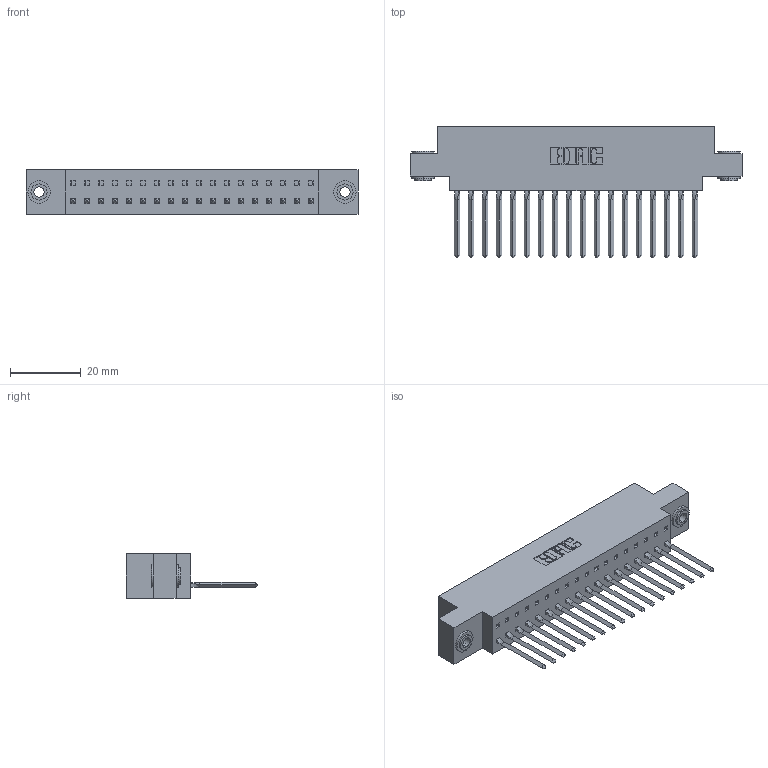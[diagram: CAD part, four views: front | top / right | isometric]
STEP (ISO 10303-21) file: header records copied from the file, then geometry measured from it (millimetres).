
FILE_DESCRIPTION (( 'STEP AP203' ), '1' );
FILE_NAME ('317-018-541-603.STEP', '2020-02-27T15:54:17', ( '' ), ( '' ), 'SwSTEP 2.0', 'SolidWorks 2016', '' );
FILE_SCHEMA (( 'CONFIG_CONTROL_DESIGN' ));
Length unit declared in the file: inch
Products named in the file (4): 317-290-002_541; 345-250-002_345-250-002-102; 317 Part_.156 Dia - TH; 317-018-541-603
Assembly tree (21 placements, depth 2):
  317-018-541-603
    317 Part_.156 Dia - TH
    317-290-002_541  x18
    345-250-002_345-250-002-102  x2
Bounding box: 94.03 x 37.34 x 12.7 mm (x, y, z)
Volume: 14530.1 mm3; surface area: 19946.5 mm2
Topology: 21 solids, 21 shells, 2876 faces, 8163 edges, 5306 vertices
Faces by surface type: plane 2300, cylinder 496, bspline 72, cone 8
Entity records: 30989 total; most frequent: CARTESIAN_POINT 6106, ORIENTED_EDGE 5370, DIRECTION 4435, EDGE_CURVE 2685, LINE 2297, VECTOR 2297, VERTEX_POINT 1780, AXIS2_PLACEMENT_3D 1069
